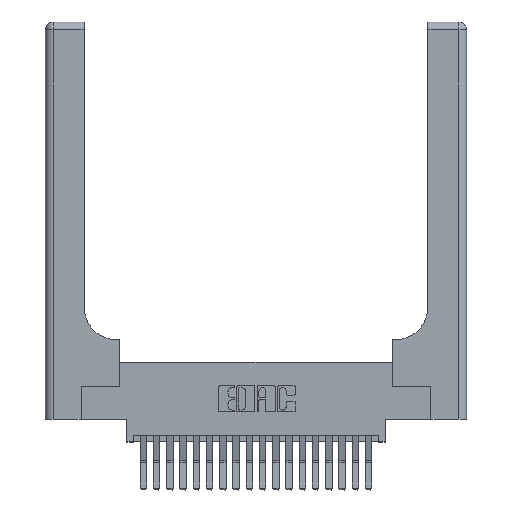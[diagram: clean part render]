
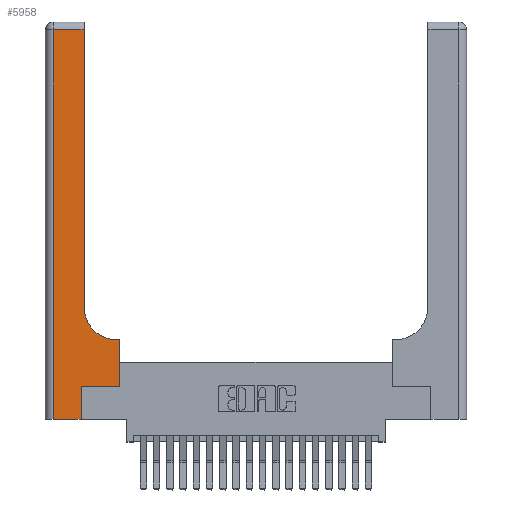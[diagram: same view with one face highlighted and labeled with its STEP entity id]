
A CAD part, top view. The second image highlights one B-rep face of the part: STEP entity #5958.
In plain terms, the highlighted planar face has unit normal (0, 0, 1).
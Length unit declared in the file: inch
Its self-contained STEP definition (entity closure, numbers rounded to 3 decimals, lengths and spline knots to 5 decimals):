
#6 = LINE ( 'NONE', #7267, #260 ) ;
#117 = VERTEX_POINT ( 'NONE', #17736 ) ;
#178 = VERTEX_POINT ( 'NONE', #21240 ) ;
#260 = VECTOR ( 'NONE', #3520, 39.37008 ) ;
#530 = VERTEX_POINT ( 'NONE', #22078 ) ;
#535 = LINE ( 'NONE', #5668, #13191 ) ;
#651 = VERTEX_POINT ( 'NONE', #10858 ) ;
#905 = CIRCLE ( 'NONE', #9159, 0.25 ) ;
#911 = DIRECTION ( 'NONE',  ( 0., 1., 0. ) ) ;
#1252 = DIRECTION ( 'NONE',  ( 1., 0., 0. ) ) ;
#1253 = AXIS2_PLACEMENT_3D ( 'NONE', #21323, #3836, #5533 ) ;
#1439 = VECTOR ( 'NONE', #1830, 39.37008 ) ;
#1608 = VERTEX_POINT ( 'NONE', #12886 ) ;
#1830 = DIRECTION ( 'NONE',  ( 1., 0., 0. ) ) ;
#2545 = LINE ( 'NONE', #13316, #17866 ) ;
#2586 = CARTESIAN_POINT ( 'NONE',  ( 0.269, 0.25, 0.37 ) ) ;
#3520 = DIRECTION ( 'NONE',  ( 0., -1., 0. ) ) ;
#3836 = DIRECTION ( 'NONE',  ( 0., 0., -1. ) ) ;
#4667 = EDGE_CURVE ( 'NONE', #178, #651, #535, .T. ) ;
#4989 = VECTOR ( 'NONE', #11420, 39.37008 ) ;
#5111 = LINE ( 'NONE', #15037, #13834 ) ;
#5533 = DIRECTION ( 'NONE',  ( -1., 0., 0. ) ) ;
#5668 = CARTESIAN_POINT ( 'NONE',  ( 0., 2.94, 0.37 ) ) ;
#5699 = PLANE ( 'NONE',  #1253 ) ;
#5958 = ADVANCED_FACE ( 'NONE', ( #10673 ), #5699, .F. ) ;
#6085 = CARTESIAN_POINT ( 'NONE',  ( 0.5415, 0.6, 0.37 ) ) ;
#6210 = CARTESIAN_POINT ( 'NONE',  ( 0.269, 0., 0.37 ) ) ;
#6676 = DIRECTION ( 'NONE',  ( -1., 0., 0. ) ) ;
#7267 = CARTESIAN_POINT ( 'NONE',  ( 0.06, 3., 0.37 ) ) ;
#7918 = EDGE_CURVE ( 'NONE', #530, #1608, #13210, .T. ) ;
#8827 = VECTOR ( 'NONE', #12013, 39.37008 ) ;
#9159 = AXIS2_PLACEMENT_3D ( 'NONE', #14631, #12992, #1252 ) ;
#9380 = VERTEX_POINT ( 'NONE', #16114 ) ;
#9709 = CARTESIAN_POINT ( 'NONE',  ( 0.2915, 3., 0.37 ) ) ;
#10111 = ORIENTED_EDGE ( 'NONE', *, *, #4667, .T. ) ;
#10265 = ORIENTED_EDGE ( 'NONE', *, *, #14508, .T. ) ;
#10673 = FACE_OUTER_BOUND ( 'NONE', #22611, .T. ) ;
#10704 = ORIENTED_EDGE ( 'NONE', *, *, #18286, .T. ) ;
#10858 = CARTESIAN_POINT ( 'NONE',  ( 0.06, 2.94, 0.37 ) ) ;
#11286 = ORIENTED_EDGE ( 'NONE', *, *, #7918, .T. ) ;
#11420 = DIRECTION ( 'NONE',  ( 0., 1., 0. ) ) ;
#11705 = ORIENTED_EDGE ( 'NONE', *, *, #18843, .T. ) ;
#11983 = ORIENTED_EDGE ( 'NONE', *, *, #16289, .T. ) ;
#12013 = DIRECTION ( 'NONE',  ( 1., 0., 0. ) ) ;
#12199 = EDGE_CURVE ( 'NONE', #117, #13669, #5111, .T. ) ;
#12286 = EDGE_CURVE ( 'NONE', #12532, #9380, #905, .T. ) ;
#12409 = CARTESIAN_POINT ( 'NONE',  ( 0.269, 0.25, 0.37 ) ) ;
#12532 = VERTEX_POINT ( 'NONE', #6085 ) ;
#12886 = CARTESIAN_POINT ( 'NONE',  ( 0.269, 0., 0.37 ) ) ;
#12992 = DIRECTION ( 'NONE',  ( 0., 0., -1. ) ) ;
#13136 = DIRECTION ( 'NONE',  ( 0., 1., 0. ) ) ;
#13191 = VECTOR ( 'NONE', #19102, 39.37008 ) ;
#13210 = LINE ( 'NONE', #18960, #8827 ) ;
#13211 = LINE ( 'NONE', #6210, #20073 ) ;
#13316 = CARTESIAN_POINT ( 'NONE',  ( 0.2915, 0.6, 0.37 ) ) ;
#13669 = VERTEX_POINT ( 'NONE', #16952 ) ;
#13834 = VECTOR ( 'NONE', #911, 39.37008 ) ;
#14350 = LINE ( 'NONE', #12409, #1439 ) ;
#14508 = EDGE_CURVE ( 'NONE', #1608, #16235, #13211, .T. ) ;
#14631 = CARTESIAN_POINT ( 'NONE',  ( 0.5415, 0.85, 0.37 ) ) ;
#15037 = CARTESIAN_POINT ( 'NONE',  ( 0.5585, 0.25, 0.37 ) ) ;
#16114 = CARTESIAN_POINT ( 'NONE',  ( 0.2915, 0.85, 0.37 ) ) ;
#16235 = VERTEX_POINT ( 'NONE', #2586 ) ;
#16289 = EDGE_CURVE ( 'NONE', #9380, #178, #16438, .T. ) ;
#16438 = LINE ( 'NONE', #9709, #4989 ) ;
#16848 = ORIENTED_EDGE ( 'NONE', *, *, #12199, .T. ) ;
#16952 = CARTESIAN_POINT ( 'NONE',  ( 0.5585, 0.6, 0.37 ) ) ;
#17736 = CARTESIAN_POINT ( 'NONE',  ( 0.5585, 0.25, 0.37 ) ) ;
#17866 = VECTOR ( 'NONE', #6676, 39.37008 ) ;
#17972 = ORIENTED_EDGE ( 'NONE', *, *, #12286, .T. ) ;
#18286 = EDGE_CURVE ( 'NONE', #16235, #117, #14350, .T. ) ;
#18843 = EDGE_CURVE ( 'NONE', #13669, #12532, #2545, .T. ) ;
#18960 = CARTESIAN_POINT ( 'NONE',  ( 0., 0., 0.37 ) ) ;
#19046 = EDGE_CURVE ( 'NONE', #651, #530, #6, .T. ) ;
#19102 = DIRECTION ( 'NONE',  ( -1., 0., 0. ) ) ;
#20073 = VECTOR ( 'NONE', #13136, 39.37008 ) ;
#20829 = ORIENTED_EDGE ( 'NONE', *, *, #19046, .T. ) ;
#21240 = CARTESIAN_POINT ( 'NONE',  ( 0.2915, 2.94, 0.37 ) ) ;
#21323 = CARTESIAN_POINT ( 'NONE',  ( 0., 3., 0.37 ) ) ;
#22078 = CARTESIAN_POINT ( 'NONE',  ( 0.06, 0., 0.37 ) ) ;
#22611 = EDGE_LOOP ( 'NONE', ( #11983, #10111, #20829, #11286, #10265, #10704, #16848, #11705, #17972 ) ) ;
